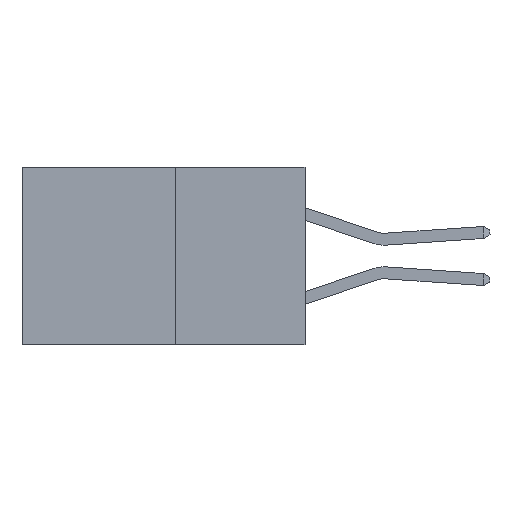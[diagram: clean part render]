
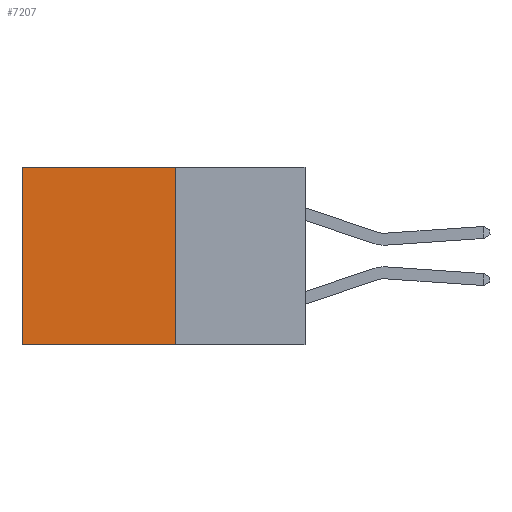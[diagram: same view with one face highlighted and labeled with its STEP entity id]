
A CAD part, left-side view. The second image highlights one B-rep face of the part: STEP entity #7207.
In plain terms, the highlighted planar face has unit normal (-1, 0, 0).
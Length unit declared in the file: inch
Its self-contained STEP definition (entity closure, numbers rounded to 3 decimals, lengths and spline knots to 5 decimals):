
#198 = DIRECTION ( 'NONE',  ( 0., 0., -1. ) ) ;
#357 = VECTOR ( 'NONE', #404, 39.37008 ) ;
#404 = DIRECTION ( 'NONE',  ( 0., 1., 0. ) ) ;
#695 = LINE ( 'NONE', #8094, #4740 ) ;
#981 = EDGE_CURVE ( 'NONE', #5499, #2604, #6968, .T. ) ;
#1120 = VERTEX_POINT ( 'NONE', #5181 ) ;
#1491 = LINE ( 'NONE', #4220, #7547 ) ;
#2204 = AXIS2_PLACEMENT_3D ( 'NONE', #9912, #7735, #3047 ) ;
#2415 = FACE_OUTER_BOUND ( 'NONE', #5921, .T. ) ;
#2466 = CARTESIAN_POINT ( 'NONE',  ( 0.277, 0.27, 0. ) ) ;
#2604 = VERTEX_POINT ( 'NONE', #7395 ) ;
#2605 = EDGE_CURVE ( 'NONE', #5499, #1120, #695, .T. ) ;
#2610 = ORIENTED_EDGE ( 'NONE', *, *, #2605, .F. ) ;
#2795 = CARTESIAN_POINT ( 'NONE',  ( 0.277, 0.27, -0.37 ) ) ;
#3047 = DIRECTION ( 'NONE',  ( 0., 0., -1. ) ) ;
#3207 = ORIENTED_EDGE ( 'NONE', *, *, #6260, .T. ) ;
#3370 = VECTOR ( 'NONE', #8217, 39.37008 ) ;
#3822 = PLANE ( 'NONE',  #2204 ) ;
#3976 = VERTEX_POINT ( 'NONE', #9716 ) ;
#3994 = ORIENTED_EDGE ( 'NONE', *, *, #5098, .F. ) ;
#4129 = ORIENTED_EDGE ( 'NONE', *, *, #981, .T. ) ;
#4220 = CARTESIAN_POINT ( 'NONE',  ( 0.277, 0.59, -0.37 ) ) ;
#4740 = VECTOR ( 'NONE', #6775, 39.37008 ) ;
#5098 = EDGE_CURVE ( 'NONE', #1120, #3976, #7555, .T. ) ;
#5181 = CARTESIAN_POINT ( 'NONE',  ( 0.277, 0.27, -0.37 ) ) ;
#5499 = VERTEX_POINT ( 'NONE', #2466 ) ;
#5921 = EDGE_LOOP ( 'NONE', ( #3207, #3994, #2610, #4129 ) ) ;
#6260 = EDGE_CURVE ( 'NONE', #2604, #3976, #1491, .T. ) ;
#6775 = DIRECTION ( 'NONE',  ( 0., 0., -1. ) ) ;
#6968 = LINE ( 'NONE', #8051, #357 ) ;
#7207 = ADVANCED_FACE ( 'NONE', ( #2415 ), #3822, .F. ) ;
#7395 = CARTESIAN_POINT ( 'NONE',  ( 0.277, 0.59, 0. ) ) ;
#7547 = VECTOR ( 'NONE', #198, 39.37008 ) ;
#7555 = LINE ( 'NONE', #2795, #3370 ) ;
#7735 = DIRECTION ( 'NONE',  ( 1., 0., 0. ) ) ;
#8051 = CARTESIAN_POINT ( 'NONE',  ( 0.277, 0.27, 0. ) ) ;
#8094 = CARTESIAN_POINT ( 'NONE',  ( 0.277, 0.27, -0.37 ) ) ;
#8217 = DIRECTION ( 'NONE',  ( 0., 1., 0. ) ) ;
#9716 = CARTESIAN_POINT ( 'NONE',  ( 0.277, 0.59, -0.37 ) ) ;
#9912 = CARTESIAN_POINT ( 'NONE',  ( 0.277, 0.27, -0.37 ) ) ;
